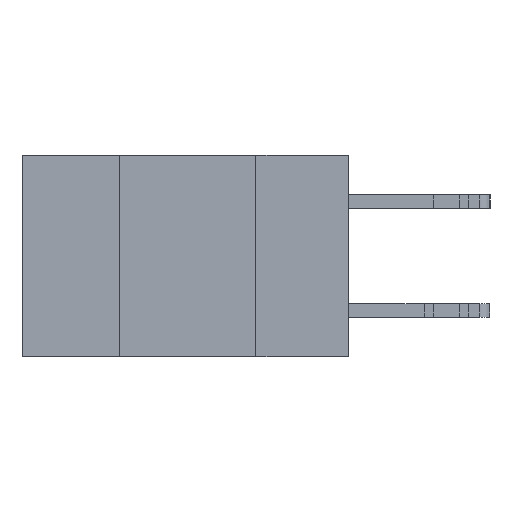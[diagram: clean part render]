
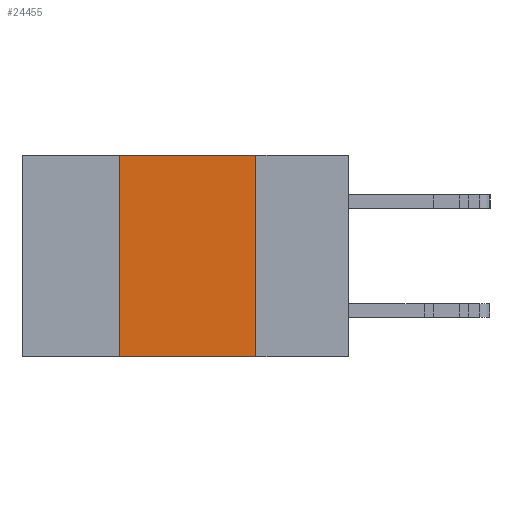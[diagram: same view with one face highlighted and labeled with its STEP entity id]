
A CAD part, left-side view. The second image highlights one B-rep face of the part: STEP entity #24455.
In plain terms, the highlighted planar face has unit normal (-1, 0, 0).
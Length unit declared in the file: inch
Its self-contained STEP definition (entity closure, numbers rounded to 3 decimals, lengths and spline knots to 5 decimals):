
#633 = DIRECTION ( 'NONE',  ( 1., 0., 0. ) ) ;
#655 = ORIENTED_EDGE ( 'NONE', *, *, #6763, .F. ) ;
#1104 = ORIENTED_EDGE ( 'NONE', *, *, #25262, .T. ) ;
#2145 = CARTESIAN_POINT ( 'NONE',  ( 0., 0.6, 0. ) ) ;
#2535 = VERTEX_POINT ( 'NONE', #20046 ) ;
#2696 = CARTESIAN_POINT ( 'NONE',  ( 0., 0.6, 0. ) ) ;
#4041 = VERTEX_POINT ( 'NONE', #16447 ) ;
#4510 = CARTESIAN_POINT ( 'NONE',  ( 0., 0.17, -0.37 ) ) ;
#4529 = EDGE_CURVE ( 'NONE', #22402, #25030, #20972, .T. ) ;
#6659 = ORIENTED_EDGE ( 'NONE', *, *, #15602, .F. ) ;
#6763 = EDGE_CURVE ( 'NONE', #4041, #22402, #7518, .T. ) ;
#7400 = ORIENTED_EDGE ( 'NONE', *, *, #4529, .F. ) ;
#7518 = LINE ( 'NONE', #24408, #15709 ) ;
#10400 = CARTESIAN_POINT ( 'NONE',  ( 0., 0.17, 0. ) ) ;
#12018 = DIRECTION ( 'NONE',  ( 0., -1., 0. ) ) ;
#12556 = DIRECTION ( 'NONE',  ( 0., 0., -1. ) ) ;
#13509 = VECTOR ( 'NONE', #12018, 39.37008 ) ;
#14920 = LINE ( 'NONE', #4510, #18149 ) ;
#15602 = EDGE_CURVE ( 'NONE', #25030, #2535, #14920, .T. ) ;
#15709 = VECTOR ( 'NONE', #20427, 39.37008 ) ;
#16447 = CARTESIAN_POINT ( 'NONE',  ( 0., 0.42, -0.37 ) ) ;
#18149 = VECTOR ( 'NONE', #25496, 39.37008 ) ;
#18448 = AXIS2_PLACEMENT_3D ( 'NONE', #2696, #633, #12556 ) ;
#20046 = CARTESIAN_POINT ( 'NONE',  ( 0., 0.17, -0.37 ) ) ;
#20243 = VECTOR ( 'NONE', #21684, 39.37008 ) ;
#20427 = DIRECTION ( 'NONE',  ( 0., 0., 1. ) ) ;
#20972 = LINE ( 'NONE', #2145, #13509 ) ;
#21285 = LINE ( 'NONE', #25777, #20243 ) ;
#21507 = PLANE ( 'NONE',  #18448 ) ;
#21684 = DIRECTION ( 'NONE',  ( 0., -1., 0. ) ) ;
#22402 = VERTEX_POINT ( 'NONE', #25183 ) ;
#23562 = FACE_OUTER_BOUND ( 'NONE', #26228, .T. ) ;
#24408 = CARTESIAN_POINT ( 'NONE',  ( 0., 0.42, -0.37 ) ) ;
#24455 = ADVANCED_FACE ( 'NONE', ( #23562 ), #21507, .F. ) ;
#25030 = VERTEX_POINT ( 'NONE', #10400 ) ;
#25183 = CARTESIAN_POINT ( 'NONE',  ( 0., 0.42, 0. ) ) ;
#25262 = EDGE_CURVE ( 'NONE', #4041, #2535, #21285, .T. ) ;
#25496 = DIRECTION ( 'NONE',  ( 0., 0., -1. ) ) ;
#25777 = CARTESIAN_POINT ( 'NONE',  ( 0., 0.6, -0.37 ) ) ;
#26228 = EDGE_LOOP ( 'NONE', ( #6659, #7400, #655, #1104 ) ) ;
